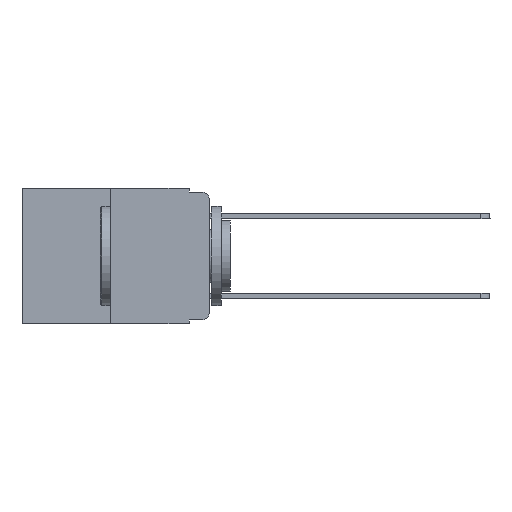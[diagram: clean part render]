
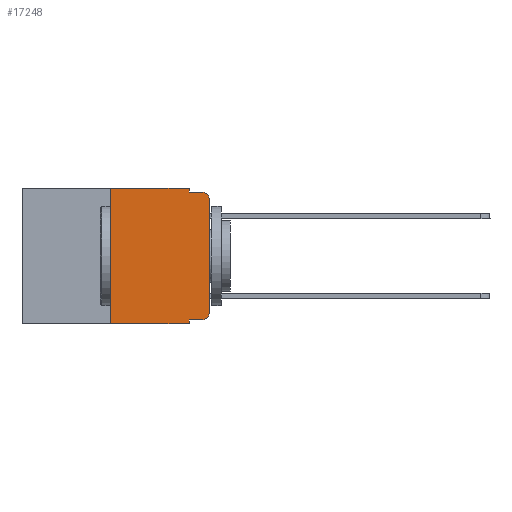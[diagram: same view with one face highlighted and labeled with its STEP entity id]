
A CAD part, left-side view. The second image highlights one B-rep face of the part: STEP entity #17248.
In plain terms, the highlighted planar face has unit normal (-1, 0, 0).
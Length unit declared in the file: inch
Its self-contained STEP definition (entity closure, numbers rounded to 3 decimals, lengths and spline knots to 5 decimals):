
#464 = ORIENTED_EDGE ( 'NONE', *, *, #677, .F. ) ;
#532 = VERTEX_POINT ( 'NONE', #17839 ) ;
#677 = EDGE_CURVE ( 'NONE', #11702, #15924, #2237, .T. ) ;
#931 = AXIS2_PLACEMENT_3D ( 'NONE', #7930, #2739, #10759 ) ;
#1131 = VECTOR ( 'NONE', #4390, 39.37008 ) ;
#1230 = VERTEX_POINT ( 'NONE', #4143 ) ;
#1604 = EDGE_CURVE ( 'NONE', #17692, #13322, #3074, .T. ) ;
#1800 = ORIENTED_EDGE ( 'NONE', *, *, #1604, .T. ) ;
#1834 = CARTESIAN_POINT ( 'NONE',  ( 0., 0.051, -0.01 ) ) ;
#1881 = AXIS2_PLACEMENT_3D ( 'NONE', #13500, #24092, #21585 ) ;
#1990 = DIRECTION ( 'NONE',  ( 0., 0., -1. ) ) ;
#2010 = VECTOR ( 'NONE', #17968, 39.37008 ) ;
#2111 = CARTESIAN_POINT ( 'NONE',  ( 0., 0.051, 0. ) ) ;
#2175 = VERTEX_POINT ( 'NONE', #13127 ) ;
#2237 = LINE ( 'NONE', #2111, #2592 ) ;
#2276 = CARTESIAN_POINT ( 'NONE',  ( 0., 0.25, 0. ) ) ;
#2304 = CIRCLE ( 'NONE', #1881, 0.02 ) ;
#2592 = VECTOR ( 'NONE', #1990, 39.37008 ) ;
#2633 = CARTESIAN_POINT ( 'NONE',  ( 0., 0.051, -0.333 ) ) ;
#2739 = DIRECTION ( 'NONE',  ( -1., 0., 0. ) ) ;
#2911 = DIRECTION ( 'NONE',  ( 0., -1., 0. ) ) ;
#3074 = CIRCLE ( 'NONE', #931, 0.02 ) ;
#3076 = EDGE_CURVE ( 'NONE', #17686, #2175, #11208, .T. ) ;
#3326 = LINE ( 'NONE', #11347, #6011 ) ;
#4072 = CARTESIAN_POINT ( 'NONE',  ( 0., 0.473, 0. ) ) ;
#4143 = CARTESIAN_POINT ( 'NONE',  ( 0., 0.25, 0. ) ) ;
#4390 = DIRECTION ( 'NONE',  ( 0., -1., 0. ) ) ;
#4496 = ORIENTED_EDGE ( 'NONE', *, *, #15324, .T. ) ;
#4772 = CARTESIAN_POINT ( 'NONE',  ( 0., 0.051, -0.333 ) ) ;
#4835 = CARTESIAN_POINT ( 'NONE',  ( 0., 0., 0. ) ) ;
#4839 = ORIENTED_EDGE ( 'NONE', *, *, #22652, .F. ) ;
#5029 = DIRECTION ( 'NONE',  ( 0., 0., -1. ) ) ;
#5126 = VECTOR ( 'NONE', #22835, 39.37008 ) ;
#5136 = ORIENTED_EDGE ( 'NONE', *, *, #6324, .F. ) ;
#5825 = ORIENTED_EDGE ( 'NONE', *, *, #23616, .F. ) ;
#6011 = VECTOR ( 'NONE', #5029, 39.37008 ) ;
#6034 = FACE_OUTER_BOUND ( 'NONE', #8466, .T. ) ;
#6104 = LINE ( 'NONE', #2276, #7884 ) ;
#6324 = EDGE_CURVE ( 'NONE', #17686, #15762, #3326, .T. ) ;
#6376 = CARTESIAN_POINT ( 'NONE',  ( 0., 0.051, -0.01 ) ) ;
#6547 = VECTOR ( 'NONE', #2911, 39.37008 ) ;
#7049 = CARTESIAN_POINT ( 'NONE',  ( 0., 0.02, -0.01 ) ) ;
#7884 = VECTOR ( 'NONE', #14405, 39.37008 ) ;
#7930 = CARTESIAN_POINT ( 'NONE',  ( 0., 0.02, -0.03 ) ) ;
#8079 = ORIENTED_EDGE ( 'NONE', *, *, #14126, .T. ) ;
#8466 = EDGE_LOOP ( 'NONE', ( #4496, #1800, #5825, #464, #15370, #4839, #8079, #5136, #11922, #15542 ) ) ;
#9283 = CARTESIAN_POINT ( 'NONE',  ( 0., 0.473, 0. ) ) ;
#10603 = LINE ( 'NONE', #24806, #5126 ) ;
#10759 = DIRECTION ( 'NONE',  ( 0., 0., -1. ) ) ;
#11141 = CARTESIAN_POINT ( 'NONE',  ( 0., 0.25, -0.343 ) ) ;
#11208 = LINE ( 'NONE', #2633, #6547 ) ;
#11347 = CARTESIAN_POINT ( 'NONE',  ( 0., 0.051, 0. ) ) ;
#11702 = VERTEX_POINT ( 'NONE', #17933 ) ;
#11922 = ORIENTED_EDGE ( 'NONE', *, *, #3076, .T. ) ;
#12101 = DIRECTION ( 'NONE',  ( 1., 0., 0. ) ) ;
#12756 = AXIS2_PLACEMENT_3D ( 'NONE', #4072, #12101, #20183 ) ;
#13127 = CARTESIAN_POINT ( 'NONE',  ( 0., 0.02, -0.333 ) ) ;
#13322 = VERTEX_POINT ( 'NONE', #7049 ) ;
#13500 = CARTESIAN_POINT ( 'NONE',  ( 0., 0.02, -0.313 ) ) ;
#14126 = EDGE_CURVE ( 'NONE', #19479, #15762, #10603, .T. ) ;
#14405 = DIRECTION ( 'NONE',  ( 0., 0., 1. ) ) ;
#15324 = EDGE_CURVE ( 'NONE', #532, #17692, #16212, .T. ) ;
#15370 = ORIENTED_EDGE ( 'NONE', *, *, #22567, .F. ) ;
#15542 = ORIENTED_EDGE ( 'NONE', *, *, #20118, .T. ) ;
#15762 = VERTEX_POINT ( 'NONE', #15808 ) ;
#15808 = CARTESIAN_POINT ( 'NONE',  ( 0., 0.051, -0.343 ) ) ;
#15924 = VERTEX_POINT ( 'NONE', #6376 ) ;
#16212 = LINE ( 'NONE', #4835, #19888 ) ;
#17248 = ADVANCED_FACE ( 'NONE', ( #6034 ), #22173, .F. ) ;
#17686 = VERTEX_POINT ( 'NONE', #4772 ) ;
#17692 = VERTEX_POINT ( 'NONE', #25008 ) ;
#17839 = CARTESIAN_POINT ( 'NONE',  ( 0., 0., -0.313 ) ) ;
#17933 = CARTESIAN_POINT ( 'NONE',  ( 0., 0.051, 0. ) ) ;
#17968 = DIRECTION ( 'NONE',  ( 0., -1., 0. ) ) ;
#19479 = VERTEX_POINT ( 'NONE', #11141 ) ;
#19888 = VECTOR ( 'NONE', #23090, 39.37008 ) ;
#20118 = EDGE_CURVE ( 'NONE', #2175, #532, #2304, .T. ) ;
#20183 = DIRECTION ( 'NONE',  ( 0., 0., -1. ) ) ;
#21585 = DIRECTION ( 'NONE',  ( 0., 0., -1. ) ) ;
#21928 = LINE ( 'NONE', #1834, #2010 ) ;
#22173 = PLANE ( 'NONE',  #12756 ) ;
#22567 = EDGE_CURVE ( 'NONE', #1230, #11702, #25846, .T. ) ;
#22652 = EDGE_CURVE ( 'NONE', #19479, #1230, #6104, .T. ) ;
#22835 = DIRECTION ( 'NONE',  ( 0., -1., 0. ) ) ;
#23090 = DIRECTION ( 'NONE',  ( 0., 0., 1. ) ) ;
#23616 = EDGE_CURVE ( 'NONE', #15924, #13322, #21928, .T. ) ;
#24092 = DIRECTION ( 'NONE',  ( -1., 0., 0. ) ) ;
#24806 = CARTESIAN_POINT ( 'NONE',  ( 0., 0.473, -0.343 ) ) ;
#25008 = CARTESIAN_POINT ( 'NONE',  ( 0., 0., -0.03 ) ) ;
#25846 = LINE ( 'NONE', #9283, #1131 ) ;
